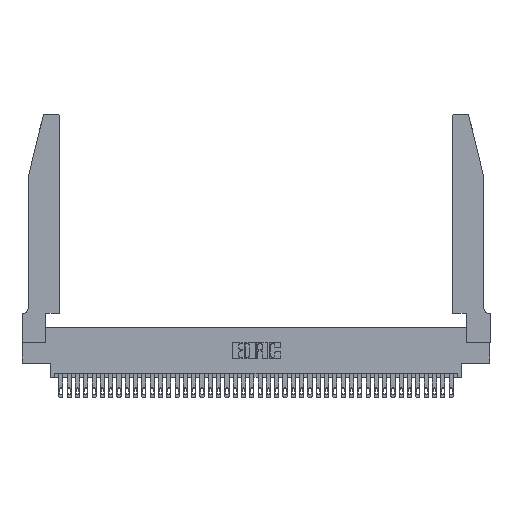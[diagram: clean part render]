
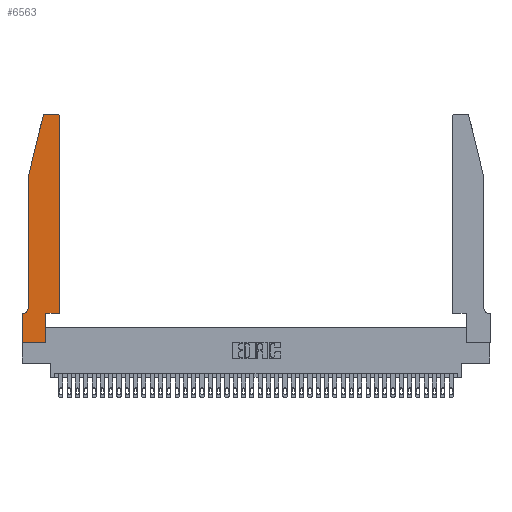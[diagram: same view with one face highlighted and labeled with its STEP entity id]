
A CAD part, top view. The second image highlights one B-rep face of the part: STEP entity #6563.
In plain terms, the highlighted planar face has unit normal (0, 0, 1).
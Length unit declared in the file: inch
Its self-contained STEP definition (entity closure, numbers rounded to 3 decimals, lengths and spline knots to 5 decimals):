
#414 = DIRECTION ( 'NONE',  ( 0., 0., 1. ) ) ;
#1428 = LINE ( 'NONE', #20652, #31674 ) ;
#1679 = DIRECTION ( 'NONE',  ( -0.239, -0.971, 0. ) ) ;
#4214 = CARTESIAN_POINT ( 'NONE',  ( 0.0055, 0.35, 0.37 ) ) ;
#4954 = CARTESIAN_POINT ( 'NONE',  ( 0.0755, 2., 0.37 ) ) ;
#5261 = VERTEX_POINT ( 'NONE', #36077 ) ;
#5969 = VECTOR ( 'NONE', #17330, 39.37008 ) ;
#6563 = ADVANCED_FACE ( 'NONE', ( #36661 ), #7151, .T. ) ;
#6677 = LINE ( 'NONE', #40936, #14756 ) ;
#7090 = LINE ( 'NONE', #4954, #24724 ) ;
#7096 = ORIENTED_EDGE ( 'NONE', *, *, #27637, .T. ) ;
#7107 = VERTEX_POINT ( 'NONE', #28694 ) ;
#7151 = PLANE ( 'NONE',  #7178 ) ;
#7178 = AXIS2_PLACEMENT_3D ( 'NONE', #10260, #414, #9852 ) ;
#7374 = DIRECTION ( 'NONE',  ( -1., 0., 0. ) ) ;
#7466 = DIRECTION ( 'NONE',  ( 1., 0., 0. ) ) ;
#8418 = ORIENTED_EDGE ( 'NONE', *, *, #38017, .T. ) ;
#8967 = CARTESIAN_POINT ( 'NONE',  ( 0.2605, 2.75, 0.37 ) ) ;
#9831 = CARTESIAN_POINT ( 'NONE',  ( 0.4205, 2.75, 0.37 ) ) ;
#9852 = DIRECTION ( 'NONE',  ( 1., 0., 0. ) ) ;
#10260 = CARTESIAN_POINT ( 'NONE',  ( 0., 0.35, 0.37 ) ) ;
#10303 = CIRCLE ( 'NONE', #28221, 0.03 ) ;
#10402 = EDGE_CURVE ( 'NONE', #16792, #28788, #39810, .T. ) ;
#10565 = EDGE_LOOP ( 'NONE', ( #16208, #8418, #7096, #11112, #39493, #35953, #14834, #17192, #21237, #33521, #28160, #18146 ) ) ;
#10647 = DIRECTION ( 'NONE',  ( 0., 0., 1. ) ) ;
#10767 = CARTESIAN_POINT ( 'NONE',  ( 0.0755, 0.35, 0.37 ) ) ;
#11008 = VERTEX_POINT ( 'NONE', #31902 ) ;
#11112 = ORIENTED_EDGE ( 'NONE', *, *, #24848, .T. ) ;
#11519 = CARTESIAN_POINT ( 'NONE',  ( 0.2865, 0.35, 0.37 ) ) ;
#11999 = EDGE_CURVE ( 'NONE', #20312, #16792, #6677, .T. ) ;
#12027 = VECTOR ( 'NONE', #37682, 39.37008 ) ;
#13122 = VERTEX_POINT ( 'NONE', #4214 ) ;
#13128 = LINE ( 'NONE', #10767, #24692 ) ;
#13240 = CIRCLE ( 'NONE', #18423, 0.03 ) ;
#13916 = DIRECTION ( 'NONE',  ( 1., 0., 0. ) ) ;
#13946 = VECTOR ( 'NONE', #16044, 39.37008 ) ;
#14401 = AXIS2_PLACEMENT_3D ( 'NONE', #19006, #22889, #29112 ) ;
#14756 = VECTOR ( 'NONE', #18070, 39.37008 ) ;
#14834 = ORIENTED_EDGE ( 'NONE', *, *, #21354, .T. ) ;
#16044 = DIRECTION ( 'NONE',  ( 0., -1., 0. ) ) ;
#16208 = ORIENTED_EDGE ( 'NONE', *, *, #31754, .T. ) ;
#16792 = VERTEX_POINT ( 'NONE', #35018 ) ;
#17192 = ORIENTED_EDGE ( 'NONE', *, *, #20015, .T. ) ;
#17330 = DIRECTION ( 'NONE',  ( 0., 1., 0. ) ) ;
#18070 = DIRECTION ( 'NONE',  ( 1., 0., 0. ) ) ;
#18146 = ORIENTED_EDGE ( 'NONE', *, *, #33924, .T. ) ;
#18423 = AXIS2_PLACEMENT_3D ( 'NONE', #33043, #10647, #13916 ) ;
#18962 = VERTEX_POINT ( 'NONE', #40531 ) ;
#19006 = CARTESIAN_POINT ( 'NONE',  ( 0.0055, 0.42, 0.37 ) ) ;
#20015 = EDGE_CURVE ( 'NONE', #22401, #11008, #1428, .T. ) ;
#20312 = VERTEX_POINT ( 'NONE', #11519 ) ;
#20347 = CARTESIAN_POINT ( 'NONE',  ( 0., 0., 0.37 ) ) ;
#20652 = CARTESIAN_POINT ( 'NONE',  ( 0., 0., 0.37 ) ) ;
#21011 = CARTESIAN_POINT ( 'NONE',  ( 0.0755, 2., 0.37 ) ) ;
#21033 = CARTESIAN_POINT ( 'NONE',  ( 0.4505, 2.72, 0.37 ) ) ;
#21237 = ORIENTED_EDGE ( 'NONE', *, *, #31550, .T. ) ;
#21354 = EDGE_CURVE ( 'NONE', #39573, #22401, #41076, .T. ) ;
#22401 = VERTEX_POINT ( 'NONE', #20347 ) ;
#22889 = DIRECTION ( 'NONE',  ( 0., 0., -1. ) ) ;
#23739 = VERTEX_POINT ( 'NONE', #9831 ) ;
#24692 = VECTOR ( 'NONE', #7374, 39.37008 ) ;
#24724 = VECTOR ( 'NONE', #39949, 39.37008 ) ;
#24848 = EDGE_CURVE ( 'NONE', #18962, #35298, #7090, .T. ) ;
#25474 = EDGE_CURVE ( 'NONE', #13122, #39573, #13128, .T. ) ;
#25992 = CIRCLE ( 'NONE', #14401, 0.07 ) ;
#26775 = CARTESIAN_POINT ( 'NONE',  ( 0.284, 2.72, 0.37 ) ) ;
#27637 = EDGE_CURVE ( 'NONE', #7107, #18962, #28775, .T. ) ;
#28160 = ORIENTED_EDGE ( 'NONE', *, *, #10402, .T. ) ;
#28221 = AXIS2_PLACEMENT_3D ( 'NONE', #26775, #32970, #7466 ) ;
#28694 = CARTESIAN_POINT ( 'NONE',  ( 0.25487, 2.72718, 0.37 ) ) ;
#28775 = LINE ( 'NONE', #21011, #36282 ) ;
#28788 = VERTEX_POINT ( 'NONE', #21033 ) ;
#29112 = DIRECTION ( 'NONE',  ( -1., 0., 0. ) ) ;
#31318 = VECTOR ( 'NONE', #38462, 39.37008 ) ;
#31550 = EDGE_CURVE ( 'NONE', #11008, #20312, #34700, .T. ) ;
#31674 = VECTOR ( 'NONE', #39601, 39.37008 ) ;
#31754 = EDGE_CURVE ( 'NONE', #23739, #5261, #35169, .T. ) ;
#31902 = CARTESIAN_POINT ( 'NONE',  ( 0.2865, 0., 0.37 ) ) ;
#32970 = DIRECTION ( 'NONE',  ( 0., 0., 1. ) ) ;
#33043 = CARTESIAN_POINT ( 'NONE',  ( 0.4205, 2.72, 0.37 ) ) ;
#33521 = ORIENTED_EDGE ( 'NONE', *, *, #11999, .T. ) ;
#33924 = EDGE_CURVE ( 'NONE', #28788, #23739, #13240, .T. ) ;
#34700 = LINE ( 'NONE', #39915, #5969 ) ;
#35018 = CARTESIAN_POINT ( 'NONE',  ( 0.4505, 0.35, 0.37 ) ) ;
#35169 = LINE ( 'NONE', #8967, #12027 ) ;
#35298 = VERTEX_POINT ( 'NONE', #37944 ) ;
#35700 = CARTESIAN_POINT ( 'NONE',  ( 0., 0., 0.37 ) ) ;
#35953 = ORIENTED_EDGE ( 'NONE', *, *, #25474, .T. ) ;
#36077 = CARTESIAN_POINT ( 'NONE',  ( 0.284, 2.75, 0.37 ) ) ;
#36282 = VECTOR ( 'NONE', #1679, 39.37008 ) ;
#36661 = FACE_OUTER_BOUND ( 'NONE', #10565, .T. ) ;
#37166 = EDGE_CURVE ( 'NONE', #35298, #13122, #25992, .T. ) ;
#37682 = DIRECTION ( 'NONE',  ( -1., 0., 0. ) ) ;
#37944 = CARTESIAN_POINT ( 'NONE',  ( 0.0755, 0.42, 0.37 ) ) ;
#38017 = EDGE_CURVE ( 'NONE', #5261, #7107, #10303, .T. ) ;
#38462 = DIRECTION ( 'NONE',  ( 0., 1., 0. ) ) ;
#39392 = CARTESIAN_POINT ( 'NONE',  ( 0., 0.35, 0.37 ) ) ;
#39493 = ORIENTED_EDGE ( 'NONE', *, *, #37166, .T. ) ;
#39573 = VERTEX_POINT ( 'NONE', #39392 ) ;
#39601 = DIRECTION ( 'NONE',  ( 1., 0., 0. ) ) ;
#39810 = LINE ( 'NONE', #41418, #31318 ) ;
#39915 = CARTESIAN_POINT ( 'NONE',  ( 0.2865, 0.35, 0.37 ) ) ;
#39949 = DIRECTION ( 'NONE',  ( 0., -1., 0. ) ) ;
#40531 = CARTESIAN_POINT ( 'NONE',  ( 0.0755, 2., 0.37 ) ) ;
#40936 = CARTESIAN_POINT ( 'NONE',  ( 0.4505, 0.35, 0.37 ) ) ;
#41076 = LINE ( 'NONE', #35700, #13946 ) ;
#41418 = CARTESIAN_POINT ( 'NONE',  ( 0.4505, 0.35, 0.37 ) ) ;
